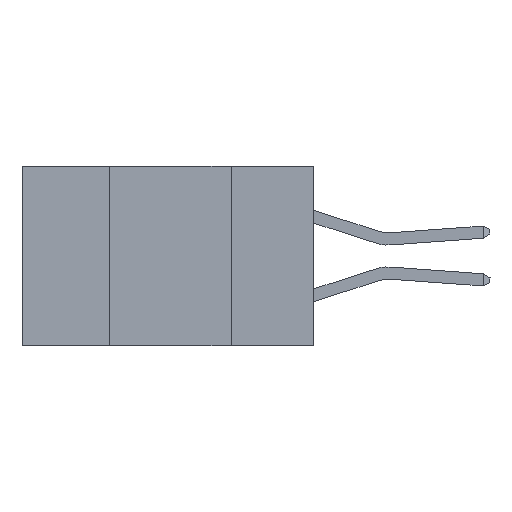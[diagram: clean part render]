
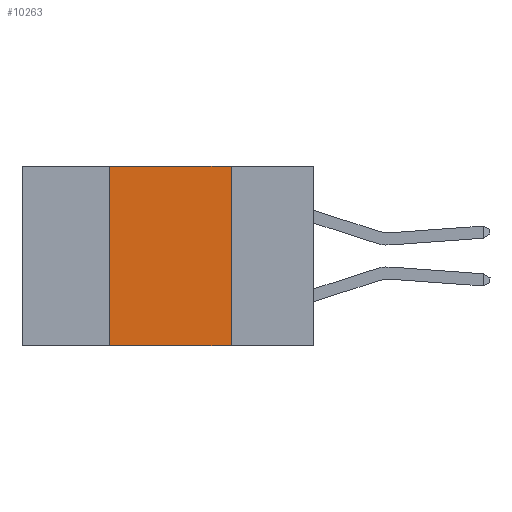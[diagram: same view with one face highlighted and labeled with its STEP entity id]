
A CAD part, left-side view. The second image highlights one B-rep face of the part: STEP entity #10263.
In plain terms, the highlighted planar face has unit normal (-1, 0, 0).
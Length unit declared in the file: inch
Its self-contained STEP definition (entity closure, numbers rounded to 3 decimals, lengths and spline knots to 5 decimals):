
#1491 = FACE_OUTER_BOUND ( 'NONE', #7743, .T. ) ;
#2487 = LINE ( 'NONE', #2611, #8029 ) ;
#2576 = ORIENTED_EDGE ( 'NONE', *, *, #7527, .F. ) ;
#2611 = CARTESIAN_POINT ( 'NONE',  ( 0., 0.42, 0. ) ) ;
#2623 = VERTEX_POINT ( 'NONE', #13900 ) ;
#3536 = CARTESIAN_POINT ( 'NONE',  ( 0., 0.17, 0. ) ) ;
#3627 = EDGE_CURVE ( 'NONE', #14712, #9601, #2487, .T. ) ;
#4059 = DIRECTION ( 'NONE',  ( 1., 0., 0. ) ) ;
#5052 = VECTOR ( 'NONE', #8059, 39.37008 ) ;
#5613 = LINE ( 'NONE', #6038, #5052 ) ;
#6038 = CARTESIAN_POINT ( 'NONE',  ( 0., 0.6, 0. ) ) ;
#7454 = PLANE ( 'NONE',  #19165 ) ;
#7527 = EDGE_CURVE ( 'NONE', #2623, #13110, #13598, .T. ) ;
#7743 = EDGE_LOOP ( 'NONE', ( #2576, #11327, #16692, #7877 ) ) ;
#7877 = ORIENTED_EDGE ( 'NONE', *, *, #15432, .T. ) ;
#8029 = VECTOR ( 'NONE', #19753, 39.37008 ) ;
#8059 = DIRECTION ( 'NONE',  ( 0., -1., 0. ) ) ;
#8848 = DIRECTION ( 'NONE',  ( 0., -1., 0. ) ) ;
#9231 = EDGE_CURVE ( 'NONE', #9601, #2623, #5613, .T. ) ;
#9312 = LINE ( 'NONE', #23003, #17405 ) ;
#9587 = CARTESIAN_POINT ( 'NONE',  ( 0., 0.17, -0.37 ) ) ;
#9601 = VERTEX_POINT ( 'NONE', #10313 ) ;
#10263 = ADVANCED_FACE ( 'NONE', ( #1491 ), #7454, .F. ) ;
#10313 = CARTESIAN_POINT ( 'NONE',  ( 0., 0.42, 0. ) ) ;
#11327 = ORIENTED_EDGE ( 'NONE', *, *, #9231, .F. ) ;
#13110 = VERTEX_POINT ( 'NONE', #9587 ) ;
#13598 = LINE ( 'NONE', #3536, #19684 ) ;
#13900 = CARTESIAN_POINT ( 'NONE',  ( 0., 0.17, 0. ) ) ;
#14712 = VERTEX_POINT ( 'NONE', #17326 ) ;
#15432 = EDGE_CURVE ( 'NONE', #14712, #13110, #9312, .T. ) ;
#16477 = DIRECTION ( 'NONE',  ( 0., 0., -1. ) ) ;
#16692 = ORIENTED_EDGE ( 'NONE', *, *, #3627, .F. ) ;
#16973 = DIRECTION ( 'NONE',  ( 0., 0., -1. ) ) ;
#17326 = CARTESIAN_POINT ( 'NONE',  ( 0., 0.42, -0.37 ) ) ;
#17405 = VECTOR ( 'NONE', #8848, 39.37008 ) ;
#19165 = AXIS2_PLACEMENT_3D ( 'NONE', #22571, #4059, #16973 ) ;
#19684 = VECTOR ( 'NONE', #16477, 39.37008 ) ;
#19753 = DIRECTION ( 'NONE',  ( 0., 0., 1. ) ) ;
#22571 = CARTESIAN_POINT ( 'NONE',  ( 0., 0.6, 0. ) ) ;
#23003 = CARTESIAN_POINT ( 'NONE',  ( 0., 0.6, -0.37 ) ) ;
